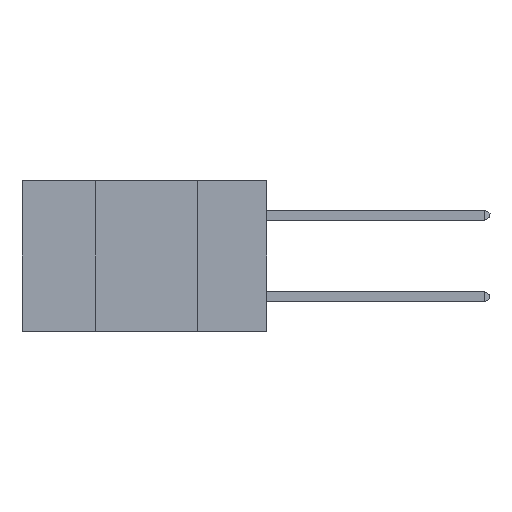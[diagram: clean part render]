
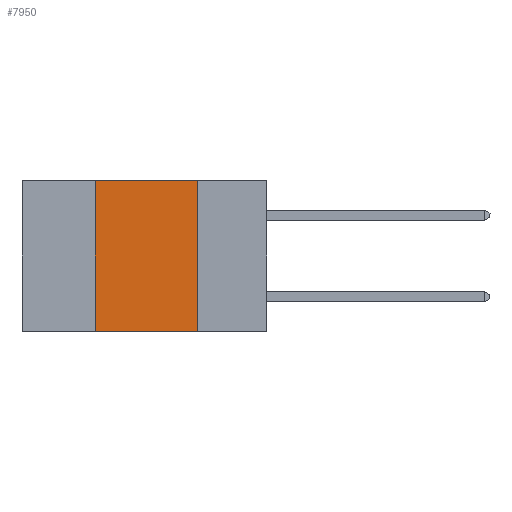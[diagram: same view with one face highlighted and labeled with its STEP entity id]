
A CAD part, left-side view. The second image highlights one B-rep face of the part: STEP entity #7950.
In plain terms, the highlighted planar face has unit normal (-1, 0, 0).
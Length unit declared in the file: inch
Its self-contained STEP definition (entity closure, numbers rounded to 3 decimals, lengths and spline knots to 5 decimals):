
#312 = ORIENTED_EDGE ( 'NONE', *, *, #6552, .T. ) ;
#853 = CARTESIAN_POINT ( 'NONE',  ( 0., 0.6, 0. ) ) ;
#1168 = PLANE ( 'NONE',  #5540 ) ;
#1494 = CARTESIAN_POINT ( 'NONE',  ( 0., 0.17, -0.37 ) ) ;
#1649 = DIRECTION ( 'NONE',  ( 0., -1., 0. ) ) ;
#2270 = DIRECTION ( 'NONE',  ( 0., 0., 1. ) ) ;
#2282 = DIRECTION ( 'NONE',  ( 0., 0., -1. ) ) ;
#2371 = CARTESIAN_POINT ( 'NONE',  ( 0., 0.42, 0. ) ) ;
#2640 = LINE ( 'NONE', #10322, #5265 ) ;
#3183 = EDGE_LOOP ( 'NONE', ( #5567, #5907, #8631, #312 ) ) ;
#4764 = VECTOR ( 'NONE', #13400, 39.37008 ) ;
#4885 = CARTESIAN_POINT ( 'NONE',  ( 0., 0.42, -0.37 ) ) ;
#5265 = VECTOR ( 'NONE', #11343, 39.37008 ) ;
#5540 = AXIS2_PLACEMENT_3D ( 'NONE', #5594, #8693, #2282 ) ;
#5567 = ORIENTED_EDGE ( 'NONE', *, *, #5897, .F. ) ;
#5594 = CARTESIAN_POINT ( 'NONE',  ( 0., 0.6, 0. ) ) ;
#5897 = EDGE_CURVE ( 'NONE', #13184, #13622, #2640, .T. ) ;
#5907 = ORIENTED_EDGE ( 'NONE', *, *, #13167, .F. ) ;
#6273 = EDGE_CURVE ( 'NONE', #12808, #11656, #9296, .T. ) ;
#6552 = EDGE_CURVE ( 'NONE', #12808, #13622, #11486, .T. ) ;
#6710 = FACE_OUTER_BOUND ( 'NONE', #3183, .T. ) ;
#7551 = LINE ( 'NONE', #853, #4764 ) ;
#7702 = CARTESIAN_POINT ( 'NONE',  ( 0., 0.42, 0. ) ) ;
#7950 = ADVANCED_FACE ( 'NONE', ( #6710 ), #1168, .F. ) ;
#8631 = ORIENTED_EDGE ( 'NONE', *, *, #6273, .F. ) ;
#8693 = DIRECTION ( 'NONE',  ( 1., 0., 0. ) ) ;
#8812 = VECTOR ( 'NONE', #1649, 39.37008 ) ;
#9090 = CARTESIAN_POINT ( 'NONE',  ( 0., 0.6, -0.37 ) ) ;
#9296 = LINE ( 'NONE', #2371, #11647 ) ;
#10322 = CARTESIAN_POINT ( 'NONE',  ( 0., 0.17, 0. ) ) ;
#11343 = DIRECTION ( 'NONE',  ( 0., 0., -1. ) ) ;
#11486 = LINE ( 'NONE', #9090, #8812 ) ;
#11504 = CARTESIAN_POINT ( 'NONE',  ( 0., 0.17, 0. ) ) ;
#11647 = VECTOR ( 'NONE', #2270, 39.37008 ) ;
#11656 = VERTEX_POINT ( 'NONE', #7702 ) ;
#12808 = VERTEX_POINT ( 'NONE', #4885 ) ;
#13167 = EDGE_CURVE ( 'NONE', #11656, #13184, #7551, .T. ) ;
#13184 = VERTEX_POINT ( 'NONE', #11504 ) ;
#13400 = DIRECTION ( 'NONE',  ( 0., -1., 0. ) ) ;
#13622 = VERTEX_POINT ( 'NONE', #1494 ) ;
